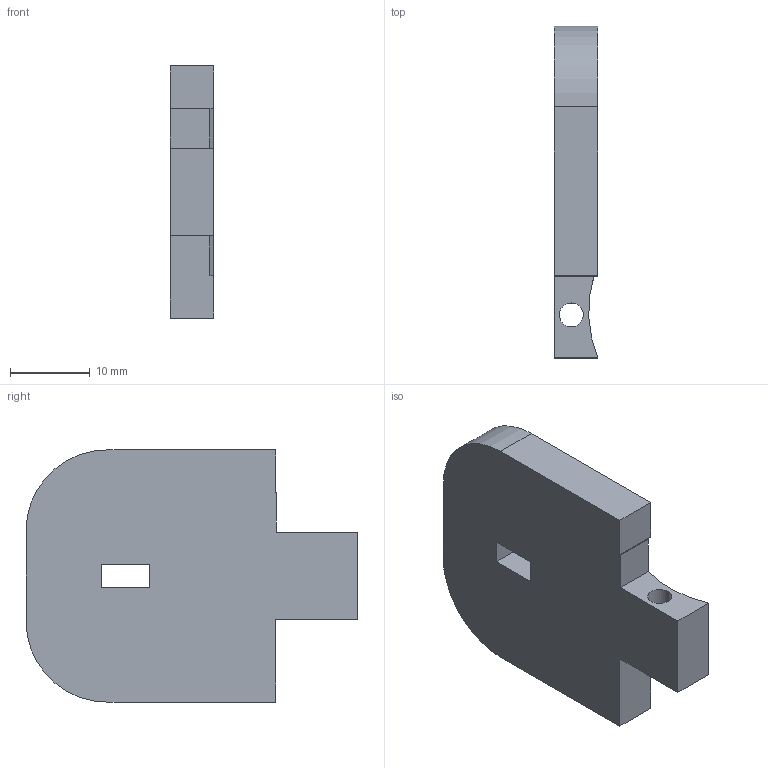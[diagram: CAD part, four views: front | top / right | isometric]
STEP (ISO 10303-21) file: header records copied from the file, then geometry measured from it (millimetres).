
FILE_DESCRIPTION (( 'STEP AP214' ), '1' );
FILE_NAME ('cover.STEP', '2013-07-25T17:03:40', ( '' ), ( '' ), 'SwSTEP 2.0', 'SolidWorks 2013', '' );
FILE_SCHEMA (( 'AUTOMOTIVE_DESIGN' ));
Length unit declared in the file: inch
Products named in the file (1): cover
Bounding box: 5.49 x 41.68 x 31.67 mm (x, y, z)
Volume: 5421.2 mm3; surface area: 3038.3 mm2
Topology: 1 solids, 1 shells, 28 faces, 77 edges, 51 vertices
Faces by surface type: plane 21, cylinder 7
Entity records: 938 total; most frequent: CARTESIAN_POINT 157, ORIENTED_EDGE 154, DIRECTION 152, EDGE_CURVE 77, VECTOR 60, LINE 60, VERTEX_POINT 51, AXIS2_PLACEMENT_3D 46
